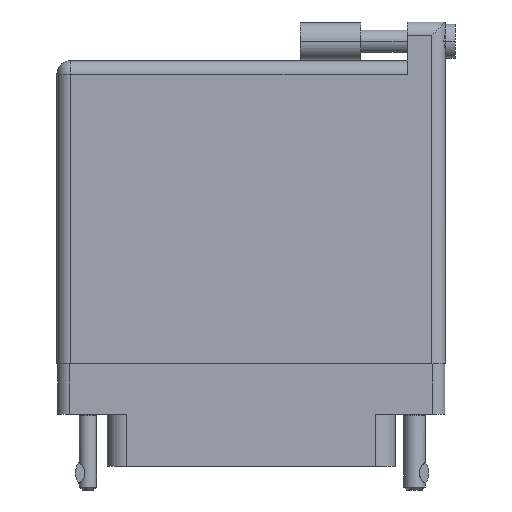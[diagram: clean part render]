
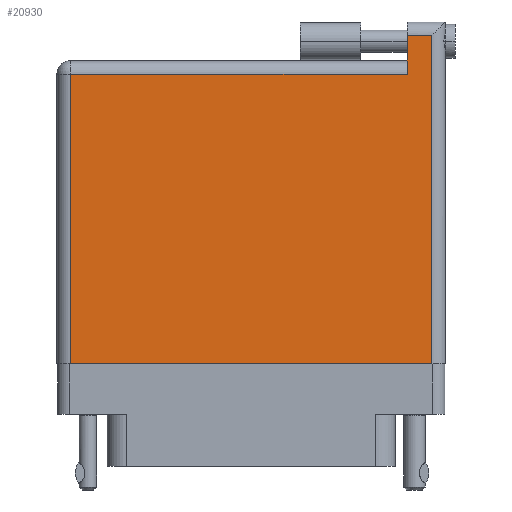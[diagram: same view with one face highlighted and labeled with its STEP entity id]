
A CAD part, front view. The second image highlights one B-rep face of the part: STEP entity #20930.
In plain terms, the highlighted face is planar.
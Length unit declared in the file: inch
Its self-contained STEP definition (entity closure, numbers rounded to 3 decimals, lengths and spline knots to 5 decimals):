
#1048 = CARTESIAN_POINT ( 'NONE',  ( 0., 1.566, 0. ) ) ;
#2259 = LINE ( 'NONE', #19462, #37439 ) ;
#3957 = AXIS2_PLACEMENT_3D ( 'NONE', #1048, #25286, #42300 ) ;
#4301 = CARTESIAN_POINT ( 'NONE',  ( 0.07, 1.496, 0. ) ) ;
#5379 = LINE ( 'NONE', #29927, #40532 ) ;
#6101 = DIRECTION ( 'NONE',  ( 0., -1., 0. ) ) ;
#6807 = CARTESIAN_POINT ( 'NONE',  ( 0.07, 0., 0. ) ) ;
#7495 = VERTEX_POINT ( 'NONE', #27154 ) ;
#8540 = VECTOR ( 'NONE', #11407, 39.37008 ) ;
#9242 = VERTEX_POINT ( 'NONE', #6807 ) ;
#9496 = DIRECTION ( 'NONE',  ( 0., -1., 0. ) ) ;
#10511 = VERTEX_POINT ( 'NONE', #34713 ) ;
#11329 = ORIENTED_EDGE ( 'NONE', *, *, #23816, .T. ) ;
#11407 = DIRECTION ( 'NONE',  ( 0., 1., 0. ) ) ;
#11461 = CARTESIAN_POINT ( 'NONE',  ( 0., 1.696, 0. ) ) ;
#14773 = EDGE_CURVE ( 'NONE', #34604, #9242, #5379, .T. ) ;
#14886 = PLANE ( 'NONE',  #3957 ) ;
#15453 = LINE ( 'NONE', #11461, #37871 ) ;
#15557 = ORIENTED_EDGE ( 'NONE', *, *, #25322, .T. ) ;
#16572 = CARTESIAN_POINT ( 'NONE',  ( 0., 1.496, 0. ) ) ;
#16800 = EDGE_CURVE ( 'NONE', #35677, #34604, #26497, .T. ) ;
#17232 = LINE ( 'NONE', #27216, #32193 ) ;
#17773 = ORIENTED_EDGE ( 'NONE', *, *, #36704, .T. ) ;
#19462 = CARTESIAN_POINT ( 'NONE',  ( 1.811, 1.766, 0. ) ) ;
#20930 = ADVANCED_FACE ( 'NONE', ( #40636 ), #14886, .F. ) ;
#22129 = CARTESIAN_POINT ( 'NONE',  ( 1.811, 1.496, 0. ) ) ;
#23816 = EDGE_CURVE ( 'NONE', #9242, #31867, #17232, .T. ) ;
#24602 = CARTESIAN_POINT ( 'NONE',  ( 1.938, 0., 0. ) ) ;
#24689 = DIRECTION ( 'NONE',  ( -1., 0., 0. ) ) ;
#24922 = CARTESIAN_POINT ( 'NONE',  ( 1.938, 1.766, 0. ) ) ;
#25286 = DIRECTION ( 'NONE',  ( 0., 0., -1. ) ) ;
#25322 = EDGE_CURVE ( 'NONE', #10511, #35677, #2259, .T. ) ;
#26497 = LINE ( 'NONE', #16572, #30830 ) ;
#26803 = EDGE_CURVE ( 'NONE', #31867, #7495, #35222, .T. ) ;
#27154 = CARTESIAN_POINT ( 'NONE',  ( 1.938, 1.696, 0. ) ) ;
#27216 = CARTESIAN_POINT ( 'NONE',  ( 0., 0., 0. ) ) ;
#28370 = ORIENTED_EDGE ( 'NONE', *, *, #26803, .T. ) ;
#28763 = EDGE_LOOP ( 'NONE', ( #11329, #28370, #17773, #15557, #29713, #36851 ) ) ;
#29713 = ORIENTED_EDGE ( 'NONE', *, *, #16800, .T. ) ;
#29927 = CARTESIAN_POINT ( 'NONE',  ( 0.07, 0., 0. ) ) ;
#30830 = VECTOR ( 'NONE', #40570, 39.37008 ) ;
#31867 = VERTEX_POINT ( 'NONE', #24602 ) ;
#32193 = VECTOR ( 'NONE', #41218, 39.37008 ) ;
#34604 = VERTEX_POINT ( 'NONE', #4301 ) ;
#34713 = CARTESIAN_POINT ( 'NONE',  ( 1.811, 1.696, 0. ) ) ;
#35222 = LINE ( 'NONE', #24922, #8540 ) ;
#35677 = VERTEX_POINT ( 'NONE', #22129 ) ;
#36704 = EDGE_CURVE ( 'NONE', #7495, #10511, #15453, .T. ) ;
#36851 = ORIENTED_EDGE ( 'NONE', *, *, #14773, .T. ) ;
#37439 = VECTOR ( 'NONE', #6101, 39.37008 ) ;
#37871 = VECTOR ( 'NONE', #24689, 39.37008 ) ;
#40532 = VECTOR ( 'NONE', #9496, 39.37008 ) ;
#40570 = DIRECTION ( 'NONE',  ( -1., 0., 0. ) ) ;
#40636 = FACE_OUTER_BOUND ( 'NONE', #28763, .T. ) ;
#41218 = DIRECTION ( 'NONE',  ( 1., 0., 0. ) ) ;
#42300 = DIRECTION ( 'NONE',  ( -1., 0., 0. ) ) ;
